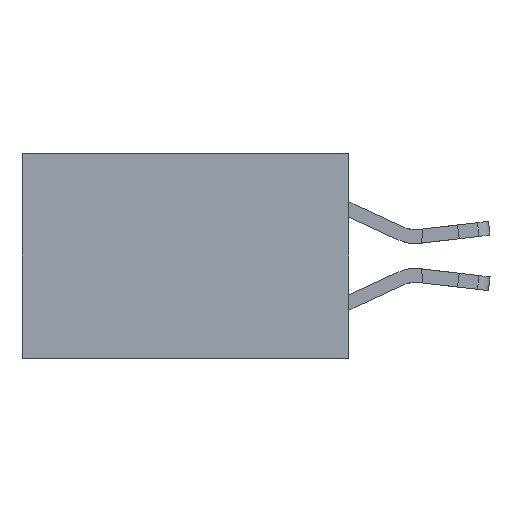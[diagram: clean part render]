
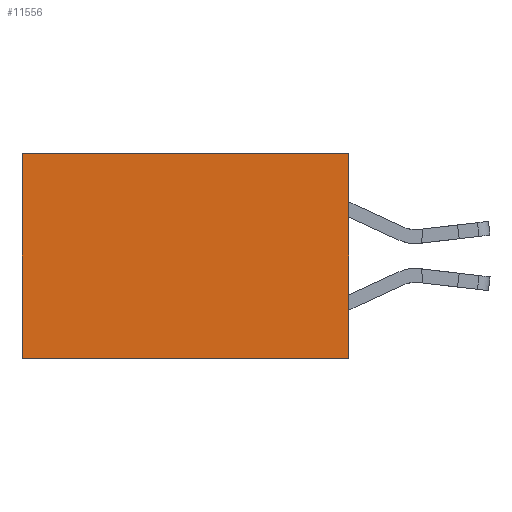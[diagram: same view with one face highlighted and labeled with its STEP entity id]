
A CAD part, left-side view. The second image highlights one B-rep face of the part: STEP entity #11556.
In plain terms, the highlighted planar face has unit normal (-1, 0, 0).
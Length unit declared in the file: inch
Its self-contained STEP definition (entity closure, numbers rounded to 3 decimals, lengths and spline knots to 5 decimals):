
#756 = CARTESIAN_POINT ( 'NONE',  ( 0.277, 0., -0.37 ) ) ;
#1235 = VECTOR ( 'NONE', #1314, 39.37008 ) ;
#1314 = DIRECTION ( 'NONE',  ( 0., 1., 0. ) ) ;
#1663 = EDGE_CURVE ( 'NONE', #13297, #2949, #15201, .T. ) ;
#1918 = AXIS2_PLACEMENT_3D ( 'NONE', #8561, #12436, #4759 ) ;
#2949 = VERTEX_POINT ( 'NONE', #6781 ) ;
#3327 = FACE_OUTER_BOUND ( 'NONE', #13509, .T. ) ;
#3383 = DIRECTION ( 'NONE',  ( 0., 0., -1. ) ) ;
#3472 = PLANE ( 'NONE',  #1918 ) ;
#4386 = CARTESIAN_POINT ( 'NONE',  ( 0.277, 0., 0. ) ) ;
#4759 = DIRECTION ( 'NONE',  ( 0., 0., -1. ) ) ;
#4911 = ORIENTED_EDGE ( 'NONE', *, *, #13822, .F. ) ;
#5653 = ORIENTED_EDGE ( 'NONE', *, *, #1663, .T. ) ;
#5846 = VERTEX_POINT ( 'NONE', #13328 ) ;
#5981 = CARTESIAN_POINT ( 'NONE',  ( 0.277, 0., -0.37 ) ) ;
#6080 = EDGE_CURVE ( 'NONE', #13815, #5846, #8108, .T. ) ;
#6781 = CARTESIAN_POINT ( 'NONE',  ( 0.277, 0.59, 0. ) ) ;
#8108 = LINE ( 'NONE', #8627, #1235 ) ;
#8561 = CARTESIAN_POINT ( 'NONE',  ( 0.277, 0., -0.37 ) ) ;
#8627 = CARTESIAN_POINT ( 'NONE',  ( 0.277, 0., -0.37 ) ) ;
#9090 = VECTOR ( 'NONE', #9151, 39.37008 ) ;
#9151 = DIRECTION ( 'NONE',  ( 0., 0., -1. ) ) ;
#9484 = LINE ( 'NONE', #11718, #9090 ) ;
#9778 = CARTESIAN_POINT ( 'NONE',  ( 0.277, 0., 0. ) ) ;
#9946 = DIRECTION ( 'NONE',  ( 0., 1., 0. ) ) ;
#11556 = ADVANCED_FACE ( 'NONE', ( #3327 ), #3472, .F. ) ;
#11718 = CARTESIAN_POINT ( 'NONE',  ( 0.277, 0.59, -0.37 ) ) ;
#12436 = DIRECTION ( 'NONE',  ( 1., 0., 0. ) ) ;
#12494 = EDGE_CURVE ( 'NONE', #2949, #5846, #9484, .T. ) ;
#12671 = ORIENTED_EDGE ( 'NONE', *, *, #12494, .T. ) ;
#13297 = VERTEX_POINT ( 'NONE', #4386 ) ;
#13328 = CARTESIAN_POINT ( 'NONE',  ( 0.277, 0.59, -0.37 ) ) ;
#13509 = EDGE_LOOP ( 'NONE', ( #12671, #16142, #4911, #5653 ) ) ;
#13815 = VERTEX_POINT ( 'NONE', #756 ) ;
#13822 = EDGE_CURVE ( 'NONE', #13297, #13815, #14302, .T. ) ;
#13910 = VECTOR ( 'NONE', #3383, 39.37008 ) ;
#14302 = LINE ( 'NONE', #5981, #13910 ) ;
#14800 = VECTOR ( 'NONE', #9946, 39.37008 ) ;
#15201 = LINE ( 'NONE', #9778, #14800 ) ;
#16142 = ORIENTED_EDGE ( 'NONE', *, *, #6080, .F. ) ;
